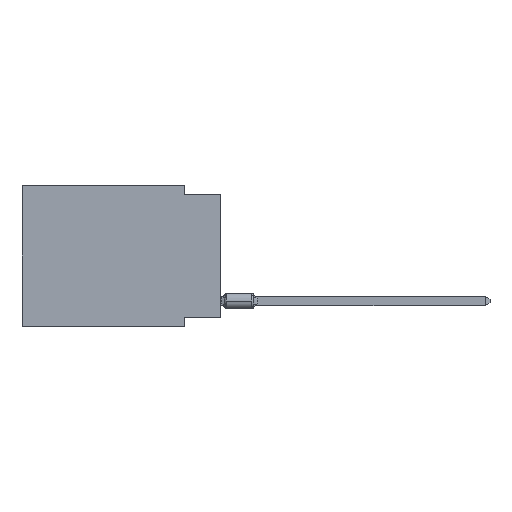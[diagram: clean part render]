
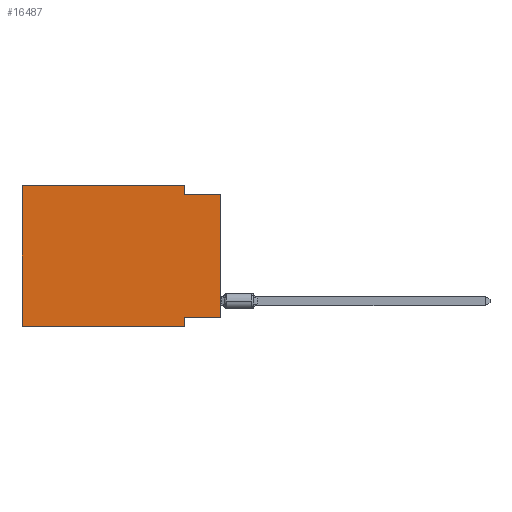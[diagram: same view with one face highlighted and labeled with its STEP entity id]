
A CAD part, left-side view. The second image highlights one B-rep face of the part: STEP entity #16487.
In plain terms, the highlighted planar face has unit normal (-1, 0, 0).
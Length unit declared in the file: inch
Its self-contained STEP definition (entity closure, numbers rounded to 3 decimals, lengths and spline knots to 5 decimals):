
#540 = CARTESIAN_POINT ( 'NONE',  ( 0., 0.55, 0. ) ) ;
#809 = VECTOR ( 'NONE', #24698, 39.37008 ) ;
#1341 = CARTESIAN_POINT ( 'NONE',  ( 0., 0., -0.025 ) ) ;
#1924 = EDGE_CURVE ( 'NONE', #20827, #33117, #9825, .T. ) ;
#2040 = VECTOR ( 'NONE', #31853, 39.37008 ) ;
#2173 = CARTESIAN_POINT ( 'NONE',  ( 0., 0.55, 0. ) ) ;
#2625 = DIRECTION ( 'NONE',  ( 0., 0., -1. ) ) ;
#2662 = DIRECTION ( 'NONE',  ( 1., 0., 0. ) ) ;
#2780 = CARTESIAN_POINT ( 'NONE',  ( 0., 0.1, 0. ) ) ;
#2967 = LINE ( 'NONE', #5671, #5249 ) ;
#3227 = VERTEX_POINT ( 'NONE', #540 ) ;
#3529 = CARTESIAN_POINT ( 'NONE',  ( 0., 0.55, 0. ) ) ;
#3734 = EDGE_CURVE ( 'NONE', #33026, #13667, #19491, .T. ) ;
#4868 = FACE_OUTER_BOUND ( 'NONE', #28034, .T. ) ;
#5249 = VECTOR ( 'NONE', #2625, 39.37008 ) ;
#5386 = VECTOR ( 'NONE', #12130, 39.37008 ) ;
#5671 = CARTESIAN_POINT ( 'NONE',  ( 0., 0.1, -0.39 ) ) ;
#6491 = AXIS2_PLACEMENT_3D ( 'NONE', #2173, #2662, #28313 ) ;
#6562 = CARTESIAN_POINT ( 'NONE',  ( 0., 0.55, 0. ) ) ;
#6965 = LINE ( 'NONE', #3529, #2040 ) ;
#7362 = CARTESIAN_POINT ( 'NONE',  ( 0., 0.1, 0. ) ) ;
#9747 = DIRECTION ( 'NONE',  ( 0., 0., -1. ) ) ;
#9825 = LINE ( 'NONE', #30555, #21957 ) ;
#9907 = LINE ( 'NONE', #7362, #12477 ) ;
#11246 = EDGE_CURVE ( 'NONE', #33117, #23886, #2967, .T. ) ;
#11470 = LINE ( 'NONE', #6562, #21452 ) ;
#11729 = CARTESIAN_POINT ( 'NONE',  ( 0., 0.1, -0.025 ) ) ;
#11881 = CARTESIAN_POINT ( 'NONE',  ( 0., 0., -0.025 ) ) ;
#11935 = LINE ( 'NONE', #17162, #23680 ) ;
#12047 = ORIENTED_EDGE ( 'NONE', *, *, #11246, .F. ) ;
#12130 = DIRECTION ( 'NONE',  ( 0., -1., 0. ) ) ;
#12477 = VECTOR ( 'NONE', #9747, 39.37008 ) ;
#13405 = EDGE_CURVE ( 'NONE', #26309, #3227, #6965, .T. ) ;
#13569 = EDGE_CURVE ( 'NONE', #3227, #31717, #11470, .T. ) ;
#13667 = VERTEX_POINT ( 'NONE', #1341 ) ;
#14462 = DIRECTION ( 'NONE',  ( 0., 0., 1. ) ) ;
#14563 = ORIENTED_EDGE ( 'NONE', *, *, #18007, .F. ) ;
#15136 = EDGE_CURVE ( 'NONE', #20827, #13667, #11935, .T. ) ;
#16378 = EDGE_CURVE ( 'NONE', #26309, #23886, #22425, .T. ) ;
#16487 = ADVANCED_FACE ( 'NONE', ( #4868 ), #22762, .F. ) ;
#17162 = CARTESIAN_POINT ( 'NONE',  ( 0., 0., 0. ) ) ;
#17185 = DIRECTION ( 'NONE',  ( 0., -1., 0. ) ) ;
#17192 = ORIENTED_EDGE ( 'NONE', *, *, #16378, .T. ) ;
#17247 = DIRECTION ( 'NONE',  ( 0., 1., 0. ) ) ;
#17391 = CARTESIAN_POINT ( 'NONE',  ( 0., 0., -0.365 ) ) ;
#18007 = EDGE_CURVE ( 'NONE', #31717, #33026, #9907, .T. ) ;
#18086 = ORIENTED_EDGE ( 'NONE', *, *, #15136, .T. ) ;
#18645 = ORIENTED_EDGE ( 'NONE', *, *, #3734, .F. ) ;
#19425 = ORIENTED_EDGE ( 'NONE', *, *, #13405, .F. ) ;
#19491 = LINE ( 'NONE', #11881, #809 ) ;
#19701 = ORIENTED_EDGE ( 'NONE', *, *, #1924, .F. ) ;
#20827 = VERTEX_POINT ( 'NONE', #17391 ) ;
#21452 = VECTOR ( 'NONE', #17185, 39.37008 ) ;
#21957 = VECTOR ( 'NONE', #17247, 39.37008 ) ;
#22425 = LINE ( 'NONE', #32370, #5386 ) ;
#22762 = PLANE ( 'NONE',  #6491 ) ;
#23336 = CARTESIAN_POINT ( 'NONE',  ( 0., 0.55, -0.39 ) ) ;
#23680 = VECTOR ( 'NONE', #14462, 39.37008 ) ;
#23886 = VERTEX_POINT ( 'NONE', #31381 ) ;
#24698 = DIRECTION ( 'NONE',  ( 0., -1., 0. ) ) ;
#25032 = CARTESIAN_POINT ( 'NONE',  ( 0., 0.1, -0.365 ) ) ;
#26309 = VERTEX_POINT ( 'NONE', #23336 ) ;
#28034 = EDGE_LOOP ( 'NONE', ( #18086, #18645, #14563, #28541, #19425, #17192, #12047, #19701 ) ) ;
#28313 = DIRECTION ( 'NONE',  ( 0., 0., -1. ) ) ;
#28541 = ORIENTED_EDGE ( 'NONE', *, *, #13569, .F. ) ;
#30555 = CARTESIAN_POINT ( 'NONE',  ( 0., 0., -0.365 ) ) ;
#31381 = CARTESIAN_POINT ( 'NONE',  ( 0., 0.1, -0.39 ) ) ;
#31717 = VERTEX_POINT ( 'NONE', #2780 ) ;
#31853 = DIRECTION ( 'NONE',  ( 0., 0., 1. ) ) ;
#32370 = CARTESIAN_POINT ( 'NONE',  ( 0., 0.55, -0.39 ) ) ;
#33026 = VERTEX_POINT ( 'NONE', #11729 ) ;
#33117 = VERTEX_POINT ( 'NONE', #25032 ) ;
